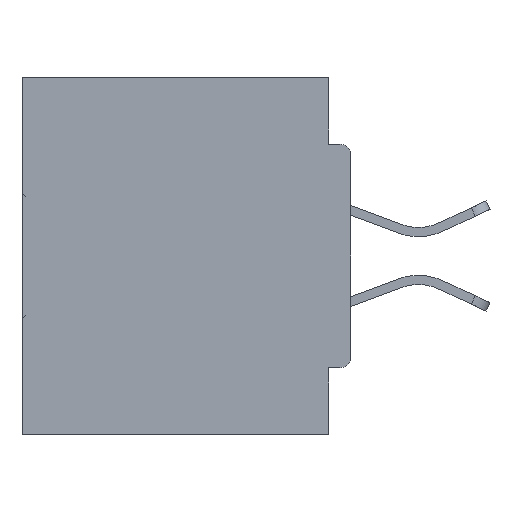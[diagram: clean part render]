
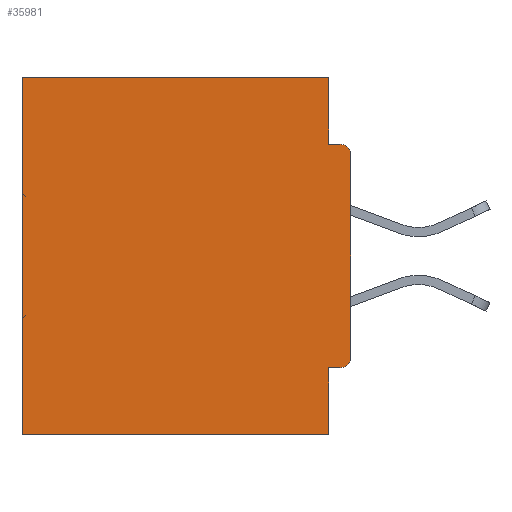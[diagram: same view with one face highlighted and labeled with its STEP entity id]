
A CAD part, left-side view. The second image highlights one B-rep face of the part: STEP entity #35981.
In plain terms, the highlighted planar face has unit normal (-1, 0, 0).
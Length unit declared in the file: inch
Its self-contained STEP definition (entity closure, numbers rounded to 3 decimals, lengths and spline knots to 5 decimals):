
#145 = DIRECTION ( 'NONE',  ( 0., 0., -1. ) ) ;
#379 = VERTEX_POINT ( 'NONE', #8954 ) ;
#733 = CARTESIAN_POINT ( 'NONE',  ( 0.298, 0., -0.3915 ) ) ;
#2083 = ORIENTED_EDGE ( 'NONE', *, *, #22284, .F. ) ;
#2258 = DIRECTION ( 'NONE',  ( -1., 0., 0. ) ) ;
#2262 = LINE ( 'NONE', #32161, #21418 ) ;
#2710 = EDGE_CURVE ( 'NONE', #39007, #29623, #15791, .T. ) ;
#2755 = CARTESIAN_POINT ( 'NONE',  ( 0.298, 0., -0.0935 ) ) ;
#3011 = ORIENTED_EDGE ( 'NONE', *, *, #19661, .T. ) ;
#3665 = VECTOR ( 'NONE', #18045, 39.37008 ) ;
#4238 = LINE ( 'NONE', #34515, #27798 ) ;
#4479 = EDGE_LOOP ( 'NONE', ( #24717, #25164, #2083, #3011, #24874, #26889, #27236, #13982, #37532, #17882 ) ) ;
#4916 = CARTESIAN_POINT ( 'NONE',  ( 0.298, 0.015, -0.4065 ) ) ;
#5384 = EDGE_CURVE ( 'NONE', #12185, #7108, #25818, .T. ) ;
#6272 = FACE_OUTER_BOUND ( 'NONE', #4479, .T. ) ;
#7108 = VERTEX_POINT ( 'NONE', #18789 ) ;
#7221 = EDGE_CURVE ( 'NONE', #36877, #39007, #35462, .T. ) ;
#7346 = EDGE_CURVE ( 'NONE', #29623, #26375, #4238, .T. ) ;
#7670 = VECTOR ( 'NONE', #27228, 39.37008 ) ;
#8464 = CARTESIAN_POINT ( 'NONE',  ( 0.298, 0., 0. ) ) ;
#8771 = DIRECTION ( 'NONE',  ( 1., 0., 0. ) ) ;
#8954 = CARTESIAN_POINT ( 'NONE',  ( 0.298, 0.031, -0.0935 ) ) ;
#11700 = LINE ( 'NONE', #39396, #21562 ) ;
#11965 = VERTEX_POINT ( 'NONE', #33478 ) ;
#12049 = EDGE_CURVE ( 'NONE', #12185, #40210, #30239, .T. ) ;
#12185 = VERTEX_POINT ( 'NONE', #40871 ) ;
#13018 = DIRECTION ( 'NONE',  ( 0., 0., -1. ) ) ;
#13102 = EDGE_CURVE ( 'NONE', #379, #7108, #43786, .T. ) ;
#13982 = ORIENTED_EDGE ( 'NONE', *, *, #7221, .F. ) ;
#14596 = AXIS2_PLACEMENT_3D ( 'NONE', #26617, #37042, #13018 ) ;
#15448 = VECTOR ( 'NONE', #21005, 39.37008 ) ;
#15600 = EDGE_CURVE ( 'NONE', #36877, #40210, #32662, .T. ) ;
#15791 = LINE ( 'NONE', #40401, #19616 ) ;
#17473 = CARTESIAN_POINT ( 'NONE',  ( 0.298, 0.46, 0. ) ) ;
#17882 = ORIENTED_EDGE ( 'NONE', *, *, #12049, .F. ) ;
#18045 = DIRECTION ( 'NONE',  ( 0., 1., 0. ) ) ;
#18743 = DIRECTION ( 'NONE',  ( 0., 0., -1. ) ) ;
#18789 = CARTESIAN_POINT ( 'NONE',  ( 0.298, 0.015, -0.0935 ) ) ;
#19392 = DIRECTION ( 'NONE',  ( 0., 0., -1. ) ) ;
#19416 = CARTESIAN_POINT ( 'NONE',  ( 0.298, 0., -0.4065 ) ) ;
#19616 = VECTOR ( 'NONE', #43445, 39.37008 ) ;
#19661 = EDGE_CURVE ( 'NONE', #11965, #31190, #26122, .T. ) ;
#21005 = DIRECTION ( 'NONE',  ( 0., 0., -1. ) ) ;
#21418 = VECTOR ( 'NONE', #145, 39.37008 ) ;
#21562 = VECTOR ( 'NONE', #18743, 39.37008 ) ;
#22284 = EDGE_CURVE ( 'NONE', #11965, #379, #2262, .T. ) ;
#22848 = AXIS2_PLACEMENT_3D ( 'NONE', #8464, #8771, #33191 ) ;
#23995 = CARTESIAN_POINT ( 'NONE',  ( 0.298, 0.46, -0.5 ) ) ;
#24717 = ORIENTED_EDGE ( 'NONE', *, *, #5384, .T. ) ;
#24874 = ORIENTED_EDGE ( 'NONE', *, *, #27805, .T. ) ;
#25164 = ORIENTED_EDGE ( 'NONE', *, *, #13102, .F. ) ;
#25818 = CIRCLE ( 'NONE', #14596, 0.015 ) ;
#26122 = LINE ( 'NONE', #32579, #3665 ) ;
#26375 = VERTEX_POINT ( 'NONE', #23995 ) ;
#26617 = CARTESIAN_POINT ( 'NONE',  ( 0.298, 0.015, -0.1085 ) ) ;
#26771 = VECTOR ( 'NONE', #33795, 39.37008 ) ;
#26889 = ORIENTED_EDGE ( 'NONE', *, *, #7346, .F. ) ;
#27062 = DIRECTION ( 'NONE',  ( 0., 1., 0. ) ) ;
#27228 = DIRECTION ( 'NONE',  ( 0., -1., 0. ) ) ;
#27236 = ORIENTED_EDGE ( 'NONE', *, *, #2710, .F. ) ;
#27798 = VECTOR ( 'NONE', #27062, 39.37008 ) ;
#27805 = EDGE_CURVE ( 'NONE', #31190, #26375, #11700, .T. ) ;
#28309 = CARTESIAN_POINT ( 'NONE',  ( 0.298, 0., 0. ) ) ;
#29612 = CARTESIAN_POINT ( 'NONE',  ( 0.298, 0.015, -0.3915 ) ) ;
#29623 = VERTEX_POINT ( 'NONE', #40636 ) ;
#29677 = CARTESIAN_POINT ( 'NONE',  ( 0.298, 0.031, -0.4065 ) ) ;
#30239 = LINE ( 'NONE', #28309, #15448 ) ;
#31190 = VERTEX_POINT ( 'NONE', #17473 ) ;
#32161 = CARTESIAN_POINT ( 'NONE',  ( 0.298, 0.031, -0.5 ) ) ;
#32579 = CARTESIAN_POINT ( 'NONE',  ( 0.298, 0., 0. ) ) ;
#32662 = CIRCLE ( 'NONE', #37260, 0.015 ) ;
#33191 = DIRECTION ( 'NONE',  ( 0., 0., -1. ) ) ;
#33478 = CARTESIAN_POINT ( 'NONE',  ( 0.298, 0.031, 0. ) ) ;
#33795 = DIRECTION ( 'NONE',  ( 0., 1., 0. ) ) ;
#34515 = CARTESIAN_POINT ( 'NONE',  ( 0.298, 0., -0.5 ) ) ;
#35462 = LINE ( 'NONE', #19416, #26771 ) ;
#35981 = ADVANCED_FACE ( 'NONE', ( #6272 ), #36414, .F. ) ;
#36414 = PLANE ( 'NONE',  #22848 ) ;
#36877 = VERTEX_POINT ( 'NONE', #4916 ) ;
#37042 = DIRECTION ( 'NONE',  ( -1., 0., 0. ) ) ;
#37260 = AXIS2_PLACEMENT_3D ( 'NONE', #29612, #2258, #19392 ) ;
#37532 = ORIENTED_EDGE ( 'NONE', *, *, #15600, .T. ) ;
#39007 = VERTEX_POINT ( 'NONE', #29677 ) ;
#39396 = CARTESIAN_POINT ( 'NONE',  ( 0.298, 0.46, 0. ) ) ;
#40210 = VERTEX_POINT ( 'NONE', #733 ) ;
#40401 = CARTESIAN_POINT ( 'NONE',  ( 0.298, 0.031, -0.5 ) ) ;
#40636 = CARTESIAN_POINT ( 'NONE',  ( 0.298, 0.031, -0.5 ) ) ;
#40871 = CARTESIAN_POINT ( 'NONE',  ( 0.298, 0., -0.1085 ) ) ;
#43445 = DIRECTION ( 'NONE',  ( 0., 0., -1. ) ) ;
#43786 = LINE ( 'NONE', #2755, #7670 ) ;
